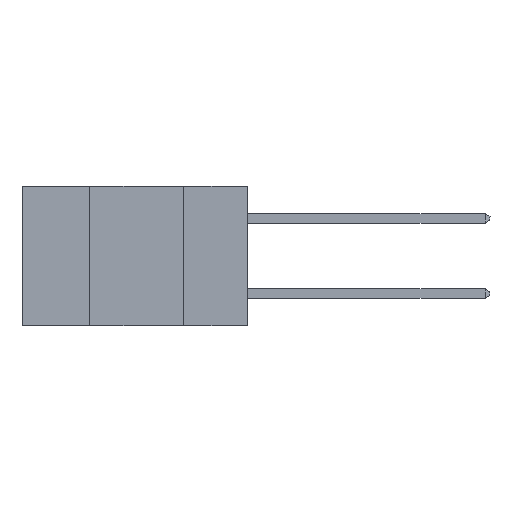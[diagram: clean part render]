
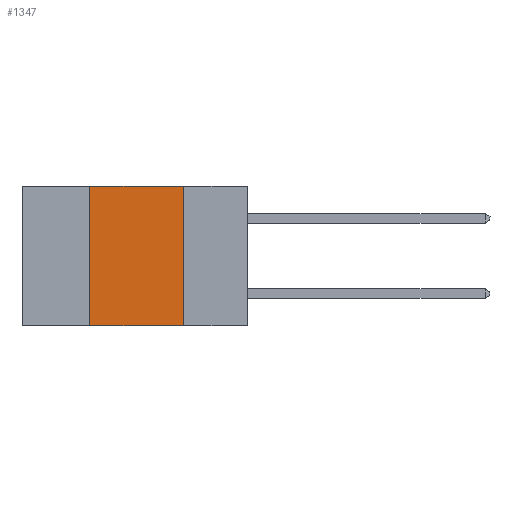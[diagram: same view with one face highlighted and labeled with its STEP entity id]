
A CAD part, left-side view. The second image highlights one B-rep face of the part: STEP entity #1347.
In plain terms, the highlighted planar face has unit normal (-1, 0, 0).
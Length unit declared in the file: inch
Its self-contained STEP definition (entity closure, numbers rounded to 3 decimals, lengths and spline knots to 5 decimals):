
#24 = EDGE_CURVE ( 'NONE', #2032, #1655, #6742, .T. ) ;
#521 = CARTESIAN_POINT ( 'NONE',  ( 0., 0.42, 0. ) ) ;
#554 = DIRECTION ( 'NONE',  ( 0., -1., 0. ) ) ;
#1082 = VECTOR ( 'NONE', #5336, 39.37008 ) ;
#1347 = ADVANCED_FACE ( 'NONE', ( #5826 ), #9370, .F. ) ;
#1371 = CARTESIAN_POINT ( 'NONE',  ( 0., 0.6, -0.37 ) ) ;
#1655 = VERTEX_POINT ( 'NONE', #10676 ) ;
#2032 = VERTEX_POINT ( 'NONE', #9772 ) ;
#2057 = VERTEX_POINT ( 'NONE', #8061 ) ;
#2343 = DIRECTION ( 'NONE',  ( 0., -1., 0. ) ) ;
#2356 = DIRECTION ( 'NONE',  ( 0., 0., -1. ) ) ;
#2674 = EDGE_CURVE ( 'NONE', #2032, #10565, #5007, .T. ) ;
#2786 = EDGE_LOOP ( 'NONE', ( #2899, #5986, #7661, #2959 ) ) ;
#2899 = ORIENTED_EDGE ( 'NONE', *, *, #10851, .F. ) ;
#2959 = ORIENTED_EDGE ( 'NONE', *, *, #24, .T. ) ;
#2966 = VECTOR ( 'NONE', #2343, 39.37008 ) ;
#3114 = DIRECTION ( 'NONE',  ( 1., 0., 0. ) ) ;
#4142 = DIRECTION ( 'NONE',  ( 0., 0., 1. ) ) ;
#4977 = LINE ( 'NONE', #8475, #6024 ) ;
#5007 = LINE ( 'NONE', #9261, #8169 ) ;
#5336 = DIRECTION ( 'NONE',  ( 0., 0., -1. ) ) ;
#5826 = FACE_OUTER_BOUND ( 'NONE', #2786, .T. ) ;
#5986 = ORIENTED_EDGE ( 'NONE', *, *, #8434, .F. ) ;
#6024 = VECTOR ( 'NONE', #554, 39.37008 ) ;
#6162 = CARTESIAN_POINT ( 'NONE',  ( 0., 0.17, -0.37 ) ) ;
#6742 = LINE ( 'NONE', #1371, #2966 ) ;
#7661 = ORIENTED_EDGE ( 'NONE', *, *, #2674, .F. ) ;
#8014 = LINE ( 'NONE', #6162, #1082 ) ;
#8061 = CARTESIAN_POINT ( 'NONE',  ( 0., 0.17, 0. ) ) ;
#8169 = VECTOR ( 'NONE', #4142, 39.37008 ) ;
#8434 = EDGE_CURVE ( 'NONE', #10565, #2057, #4977, .T. ) ;
#8475 = CARTESIAN_POINT ( 'NONE',  ( 0., 0.6, 0. ) ) ;
#8518 = AXIS2_PLACEMENT_3D ( 'NONE', #11096, #3114, #2356 ) ;
#9261 = CARTESIAN_POINT ( 'NONE',  ( 0., 0.42, -0.37 ) ) ;
#9370 = PLANE ( 'NONE',  #8518 ) ;
#9772 = CARTESIAN_POINT ( 'NONE',  ( 0., 0.42, -0.37 ) ) ;
#10565 = VERTEX_POINT ( 'NONE', #521 ) ;
#10676 = CARTESIAN_POINT ( 'NONE',  ( 0., 0.17, -0.37 ) ) ;
#10851 = EDGE_CURVE ( 'NONE', #2057, #1655, #8014, .T. ) ;
#11096 = CARTESIAN_POINT ( 'NONE',  ( 0., 0.6, 0. ) ) ;
